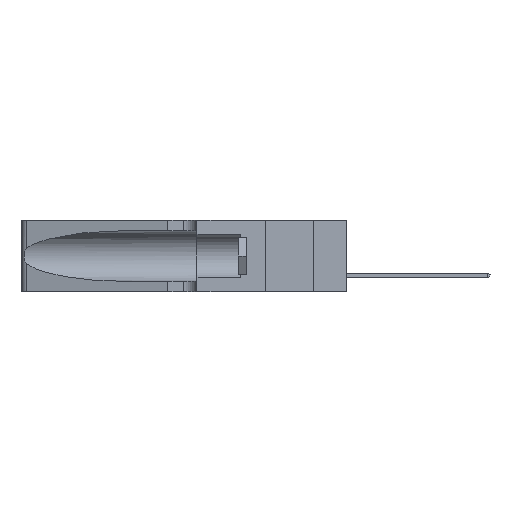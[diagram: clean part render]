
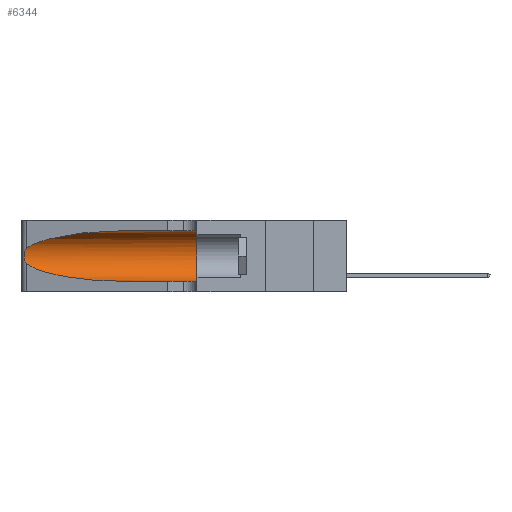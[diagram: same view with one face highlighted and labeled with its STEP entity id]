
A CAD part, left-side view. The second image highlights one B-rep face of the part: STEP entity #6344.
In plain terms, the highlighted cylindrical face has radius 3.308 mm (diameter 6.617 mm), a partial arc.
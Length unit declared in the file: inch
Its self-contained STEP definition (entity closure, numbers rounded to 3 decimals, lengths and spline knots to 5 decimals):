
#1805 = ORIENTED_EDGE ( 'NONE', *, *, #36211, .F. ) ;
#1860 = CARTESIAN_POINT ( 'NONE',  ( 0.25639, 1.23186, 0.15144 ) ) ;
#1931 = CARTESIAN_POINT ( 'NONE',  ( 0.25487, 1.22718, 0.14631 ) ) ;
#3085 = DIRECTION ( 'NONE',  ( 0., 1., 0. ) ) ;
#3282 = EDGE_LOOP ( 'NONE', ( #25657, #7501, #31673, #10774, #1805, #30139 ) ) ;
#4313 = VERTEX_POINT ( 'NONE', #9176 ) ;
#5193 = CARTESIAN_POINT ( 'NONE',  ( 0.1305, 1.61858, 0.185 ) ) ;
#5311 = DIRECTION ( 'NONE',  ( 0., -1., 0. ) ) ;
#5745 = CARTESIAN_POINT ( 'NONE',  ( 0.26018, 1.23835, 0.19895 ) ) ;
#6344 = ADVANCED_FACE ( 'NONE', ( #19147 ), #24818, .F. ) ;
#6403 = CARTESIAN_POINT ( 'NONE',  ( 0.2373, 1.15595, 0.08982 ) ) ;
#7174 = CARTESIAN_POINT ( 'NONE',  ( 0.2373, 1.15595, 0.28018 ) ) ;
#7252 = LINE ( 'NONE', #33809, #18647 ) ;
#7501 = ORIENTED_EDGE ( 'NONE', *, *, #23485, .T. ) ;
#8541 = CARTESIAN_POINT ( 'NONE',  ( 0.25854, 1.2359, 0.20912 ) ) ;
#9176 = CARTESIAN_POINT ( 'NONE',  ( 0.1305, 0.35, 0.05475 ) ) ;
#10408 = CARTESIAN_POINT ( 'NONE',  ( 0.25555, 1.22994, 0.2215 ) ) ;
#10472 = B_SPLINE_CURVE_WITH_KNOTS ( 'NONE', 3,
 ( #27516, #10408, #13186, #11231, #8541, #5745, #19674, #11341, #22787, #17439, #11455, #1860, #22257, #20400 ),
 .UNSPECIFIED., .F., .F.,
 ( 4, 2, 2, 2, 2, 2, 4 ),
 ( 0., 0.00027, 0.00053, 0.00107, 0.0016, 0.00187, 0.00214 ),
 .UNSPECIFIED. ) ;
#10534 = EDGE_CURVE ( 'NONE', #19717, #4313, #13564, .T. ) ;
#10774 = ORIENTED_EDGE ( 'NONE', *, *, #10534, .T. ) ;
#11231 = CARTESIAN_POINT ( 'NONE',  ( 0.25787, 1.23484, 0.2124 ) ) ;
#11341 = CARTESIAN_POINT ( 'NONE',  ( 0.26075, 1.23896, 0.178 ) ) ;
#11455 = CARTESIAN_POINT ( 'NONE',  ( 0.25789, 1.23486, 0.15765 ) ) ;
#11772 = EDGE_CURVE ( 'NONE', #26024, #19717, #35947, .T. ) ;
#11851 = CARTESIAN_POINT ( 'NONE',  ( 0.1305, 1.61858, 0.05475 ) ) ;
#12321 = CIRCLE ( 'NONE', #12711, 0.13025 ) ;
#12711 = AXIS2_PLACEMENT_3D ( 'NONE', #28381, #3085, #30728 ) ;
#13186 = CARTESIAN_POINT ( 'NONE',  ( 0.25639, 1.23184, 0.21858 ) ) ;
#13564 = LINE ( 'NONE', #11851, #34977 ) ;
#13857 = CARTESIAN_POINT ( 'NONE',  ( 0.1305, 0.72297, 0.31525 ) ) ;
#14297 = VERTEX_POINT ( 'NONE', #29275 ) ;
#16030 = VERTEX_POINT ( 'NONE', #26736 ) ;
#17439 = CARTESIAN_POINT ( 'NONE',  ( 0.25856, 1.23593, 0.16098 ) ) ;
#18647 = VECTOR ( 'NONE', #30894, 39.37008 ) ;
#19147 = FACE_OUTER_BOUND ( 'NONE', #3282, .T. ) ;
#19674 = CARTESIAN_POINT ( 'NONE',  ( 0.26075, 1.23896, 0.19203 ) ) ;
#19717 = VERTEX_POINT ( 'NONE', #34752 ) ;
#20197 = CARTESIAN_POINT ( 'NONE',  ( 0.25487, 1.22718, 0.14631 ) ) ;
#20271 =( BOUNDED_CURVE ( )  B_SPLINE_CURVE ( 3, ( #23907, #32454, #7174, #26735 ),
 .UNSPECIFIED., .F., .T. ) 
 B_SPLINE_CURVE_WITH_KNOTS ( ( 4, 4 ),
 ( 1.5708, 2.84003 ),
 .UNSPECIFIED. ) 
 CURVE ( )  GEOMETRIC_REPRESENTATION_ITEM ( )  RATIONAL_B_SPLINE_CURVE ( ( 1., 0.87, 0.87, 1. ) ) 
 REPRESENTATION_ITEM ( '' )  );
#20400 = CARTESIAN_POINT ( 'NONE',  ( 0.25487, 1.22718, 0.14631 ) ) ;
#22257 = CARTESIAN_POINT ( 'NONE',  ( 0.25555, 1.22993, 0.14849 ) ) ;
#22787 = CARTESIAN_POINT ( 'NONE',  ( 0.26017, 1.23833, 0.17102 ) ) ;
#23205 = DIRECTION ( 'NONE',  ( 0., -1., 0. ) ) ;
#23238 = CARTESIAN_POINT ( 'NONE',  ( 0.18966, 0.96281, 0.05475 ) ) ;
#23485 = EDGE_CURVE ( 'NONE', #14297, #26024, #10472, .T. ) ;
#23907 = CARTESIAN_POINT ( 'NONE',  ( 0.1305, 0.72297, 0.31525 ) ) ;
#24818 = CYLINDRICAL_SURFACE ( 'NONE', #33951, 0.13025 ) ;
#25657 = ORIENTED_EDGE ( 'NONE', *, *, #33239, .T. ) ;
#26024 = VERTEX_POINT ( 'NONE', #1931 ) ;
#26735 = CARTESIAN_POINT ( 'NONE',  ( 0.25487, 1.22718, 0.22369 ) ) ;
#26736 = CARTESIAN_POINT ( 'NONE',  ( 0.1305, 0.35, 0.31525 ) ) ;
#27516 = CARTESIAN_POINT ( 'NONE',  ( 0.25487, 1.22718, 0.22369 ) ) ;
#27677 = DIRECTION ( 'NONE',  ( 0., 0., -1. ) ) ;
#28381 = CARTESIAN_POINT ( 'NONE',  ( 0.1305, 0.35, 0.185 ) ) ;
#29275 = CARTESIAN_POINT ( 'NONE',  ( 0.25487, 1.22718, 0.22369 ) ) ;
#30139 = ORIENTED_EDGE ( 'NONE', *, *, #30202, .F. ) ;
#30202 = EDGE_CURVE ( 'NONE', #36106, #16030, #7252, .T. ) ;
#30728 = DIRECTION ( 'NONE',  ( 0., 0., 1. ) ) ;
#30894 = DIRECTION ( 'NONE',  ( 0., -1., 0. ) ) ;
#31673 = ORIENTED_EDGE ( 'NONE', *, *, #11772, .T. ) ;
#32454 = CARTESIAN_POINT ( 'NONE',  ( 0.18966, 0.96281, 0.31525 ) ) ;
#33239 = EDGE_CURVE ( 'NONE', #36106, #14297, #20271, .T. ) ;
#33809 = CARTESIAN_POINT ( 'NONE',  ( 0.1305, 1.61858, 0.31525 ) ) ;
#33951 = AXIS2_PLACEMENT_3D ( 'NONE', #5193, #5311, #27677 ) ;
#34468 = CARTESIAN_POINT ( 'NONE',  ( 0.1305, 0.72297, 0.05475 ) ) ;
#34752 = CARTESIAN_POINT ( 'NONE',  ( 0.1305, 0.72297, 0.05475 ) ) ;
#34977 = VECTOR ( 'NONE', #23205, 39.37008 ) ;
#35947 =( BOUNDED_CURVE ( )  B_SPLINE_CURVE ( 3, ( #20197, #6403, #23238, #34468 ),
 .UNSPECIFIED., .F., .F. ) 
 B_SPLINE_CURVE_WITH_KNOTS ( ( 4, 4 ),
 ( 3.44316, 4.71239 ),
 .UNSPECIFIED. ) 
 CURVE ( )  GEOMETRIC_REPRESENTATION_ITEM ( )  RATIONAL_B_SPLINE_CURVE ( ( 1., 0.87, 0.87, 1. ) ) 
 REPRESENTATION_ITEM ( '' )  );
#36106 = VERTEX_POINT ( 'NONE', #13857 ) ;
#36211 = EDGE_CURVE ( 'NONE', #16030, #4313, #12321, .T. ) ;
